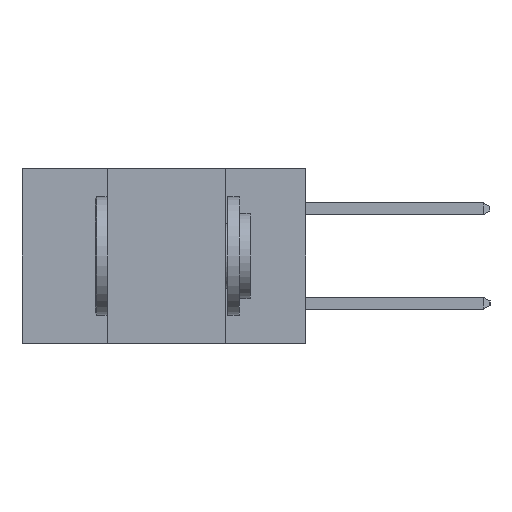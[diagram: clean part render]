
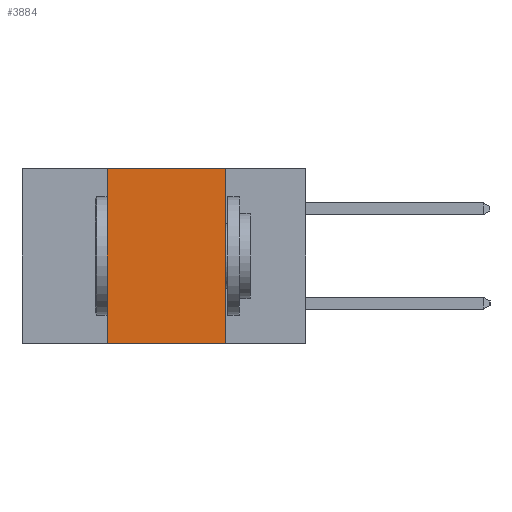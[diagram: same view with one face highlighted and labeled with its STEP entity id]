
A CAD part, left-side view. The second image highlights one B-rep face of the part: STEP entity #3884.
In plain terms, the highlighted planar face has unit normal (-1, 0, 0).
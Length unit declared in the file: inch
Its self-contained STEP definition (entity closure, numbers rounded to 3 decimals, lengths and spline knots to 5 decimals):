
#251 = CARTESIAN_POINT ( 'NONE',  ( 0., 0.6, 0. ) ) ;
#344 = CARTESIAN_POINT ( 'NONE',  ( 0., 0.17, -0.37 ) ) ;
#908 = VECTOR ( 'NONE', #8692, 39.37008 ) ;
#939 = EDGE_CURVE ( 'NONE', #7146, #7379, #1157, .T. ) ;
#1157 = LINE ( 'NONE', #1266, #908 ) ;
#1266 = CARTESIAN_POINT ( 'NONE',  ( 0., 0.6, -0.37 ) ) ;
#1372 = AXIS2_PLACEMENT_3D ( 'NONE', #4458, #6077, #5111 ) ;
#1920 = CARTESIAN_POINT ( 'NONE',  ( 0., 0.42, 0. ) ) ;
#2479 = EDGE_CURVE ( 'NONE', #7146, #7376, #6249, .T. ) ;
#2545 = ORIENTED_EDGE ( 'NONE', *, *, #939, .T. ) ;
#2770 = FACE_OUTER_BOUND ( 'NONE', #8314, .T. ) ;
#2794 = VECTOR ( 'NONE', #9773, 39.37008 ) ;
#2995 = EDGE_CURVE ( 'NONE', #7376, #4215, #8864, .T. ) ;
#3884 = ADVANCED_FACE ( 'NONE', ( #2770 ), #3947, .F. ) ;
#3947 = PLANE ( 'NONE',  #1372 ) ;
#4093 = EDGE_CURVE ( 'NONE', #4215, #7379, #6326, .T. ) ;
#4193 = VECTOR ( 'NONE', #5040, 39.37008 ) ;
#4215 = VERTEX_POINT ( 'NONE', #6202 ) ;
#4426 = ORIENTED_EDGE ( 'NONE', *, *, #4093, .F. ) ;
#4458 = CARTESIAN_POINT ( 'NONE',  ( 0., 0.6, 0. ) ) ;
#5040 = DIRECTION ( 'NONE',  ( 0., 0., 1. ) ) ;
#5043 = CARTESIAN_POINT ( 'NONE',  ( 0., 0.42, -0.37 ) ) ;
#5111 = DIRECTION ( 'NONE',  ( 0., 0., -1. ) ) ;
#5226 = DIRECTION ( 'NONE',  ( 0., 0., -1. ) ) ;
#6077 = DIRECTION ( 'NONE',  ( 1., 0., 0. ) ) ;
#6202 = CARTESIAN_POINT ( 'NONE',  ( 0., 0.17, 0. ) ) ;
#6249 = LINE ( 'NONE', #5043, #4193 ) ;
#6326 = LINE ( 'NONE', #6801, #8107 ) ;
#6466 = ORIENTED_EDGE ( 'NONE', *, *, #2995, .F. ) ;
#6801 = CARTESIAN_POINT ( 'NONE',  ( 0., 0.17, -0.37 ) ) ;
#7146 = VERTEX_POINT ( 'NONE', #9775 ) ;
#7376 = VERTEX_POINT ( 'NONE', #1920 ) ;
#7379 = VERTEX_POINT ( 'NONE', #344 ) ;
#8107 = VECTOR ( 'NONE', #5226, 39.37008 ) ;
#8314 = EDGE_LOOP ( 'NONE', ( #4426, #6466, #8446, #2545 ) ) ;
#8446 = ORIENTED_EDGE ( 'NONE', *, *, #2479, .F. ) ;
#8692 = DIRECTION ( 'NONE',  ( 0., -1., 0. ) ) ;
#8864 = LINE ( 'NONE', #251, #2794 ) ;
#9773 = DIRECTION ( 'NONE',  ( 0., -1., 0. ) ) ;
#9775 = CARTESIAN_POINT ( 'NONE',  ( 0., 0.42, -0.37 ) ) ;
